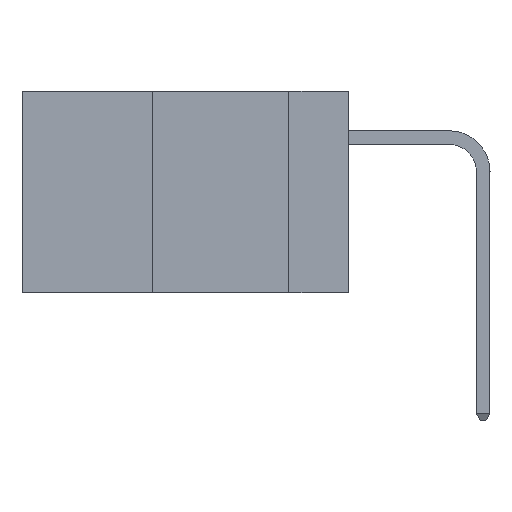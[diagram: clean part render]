
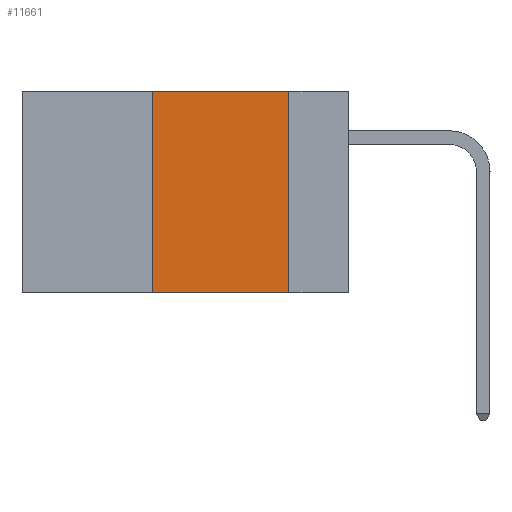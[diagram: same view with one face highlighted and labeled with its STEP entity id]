
A CAD part, left-side view. The second image highlights one B-rep face of the part: STEP entity #11661.
In plain terms, the highlighted planar face has unit normal (-1, 0, 0).
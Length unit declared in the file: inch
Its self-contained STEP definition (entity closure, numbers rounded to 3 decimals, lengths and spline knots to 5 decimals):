
#330 = PLANE ( 'NONE',  #6592 ) ;
#332 = FACE_OUTER_BOUND ( 'NONE', #3287, .T. ) ;
#512 = EDGE_CURVE ( 'NONE', #9278, #11222, #6470, .T. ) ;
#570 = DIRECTION ( 'NONE',  ( 0., -1., 0. ) ) ;
#922 = ORIENTED_EDGE ( 'NONE', *, *, #5839, .T. ) ;
#1019 = ORIENTED_EDGE ( 'NONE', *, *, #512, .F. ) ;
#1506 = DIRECTION ( 'NONE',  ( 1., 0., 0. ) ) ;
#1739 = VECTOR ( 'NONE', #11606, 39.37008 ) ;
#2347 = ORIENTED_EDGE ( 'NONE', *, *, #12557, .F. ) ;
#2501 = ORIENTED_EDGE ( 'NONE', *, *, #10066, .F. ) ;
#3009 = LINE ( 'NONE', #7037, #8072 ) ;
#3050 = LINE ( 'NONE', #6890, #3441 ) ;
#3287 = EDGE_LOOP ( 'NONE', ( #1019, #2501, #2347, #922 ) ) ;
#3441 = VECTOR ( 'NONE', #570, 39.37008 ) ;
#4839 = CARTESIAN_POINT ( 'NONE',  ( 0., 0.11, -0.37 ) ) ;
#5839 = EDGE_CURVE ( 'NONE', #11876, #11222, #3009, .T. ) ;
#6007 = DIRECTION ( 'NONE',  ( 0., 0., -1. ) ) ;
#6050 = CARTESIAN_POINT ( 'NONE',  ( 0., 0.11, 0. ) ) ;
#6164 = VECTOR ( 'NONE', #6007, 39.37008 ) ;
#6470 = LINE ( 'NONE', #6050, #6164 ) ;
#6592 = AXIS2_PLACEMENT_3D ( 'NONE', #10495, #1506, #8708 ) ;
#6841 = CARTESIAN_POINT ( 'NONE',  ( 0., 0.36, 0. ) ) ;
#6890 = CARTESIAN_POINT ( 'NONE',  ( 0., 0.6, 0. ) ) ;
#7037 = CARTESIAN_POINT ( 'NONE',  ( 0., 0.6, -0.37 ) ) ;
#7053 = DIRECTION ( 'NONE',  ( 0., -1., 0. ) ) ;
#7245 = LINE ( 'NONE', #8992, #1739 ) ;
#8072 = VECTOR ( 'NONE', #7053, 39.37008 ) ;
#8708 = DIRECTION ( 'NONE',  ( 0., 0., -1. ) ) ;
#8992 = CARTESIAN_POINT ( 'NONE',  ( 0., 0.36, 0. ) ) ;
#9278 = VERTEX_POINT ( 'NONE', #12234 ) ;
#10066 = EDGE_CURVE ( 'NONE', #12245, #9278, #3050, .T. ) ;
#10495 = CARTESIAN_POINT ( 'NONE',  ( 0., 0.6, 0. ) ) ;
#11222 = VERTEX_POINT ( 'NONE', #4839 ) ;
#11606 = DIRECTION ( 'NONE',  ( 0., 0., 1. ) ) ;
#11661 = ADVANCED_FACE ( 'NONE', ( #332 ), #330, .F. ) ;
#11687 = CARTESIAN_POINT ( 'NONE',  ( 0., 0.36, -0.37 ) ) ;
#11876 = VERTEX_POINT ( 'NONE', #11687 ) ;
#12234 = CARTESIAN_POINT ( 'NONE',  ( 0., 0.11, 0. ) ) ;
#12245 = VERTEX_POINT ( 'NONE', #6841 ) ;
#12557 = EDGE_CURVE ( 'NONE', #11876, #12245, #7245, .T. ) ;
